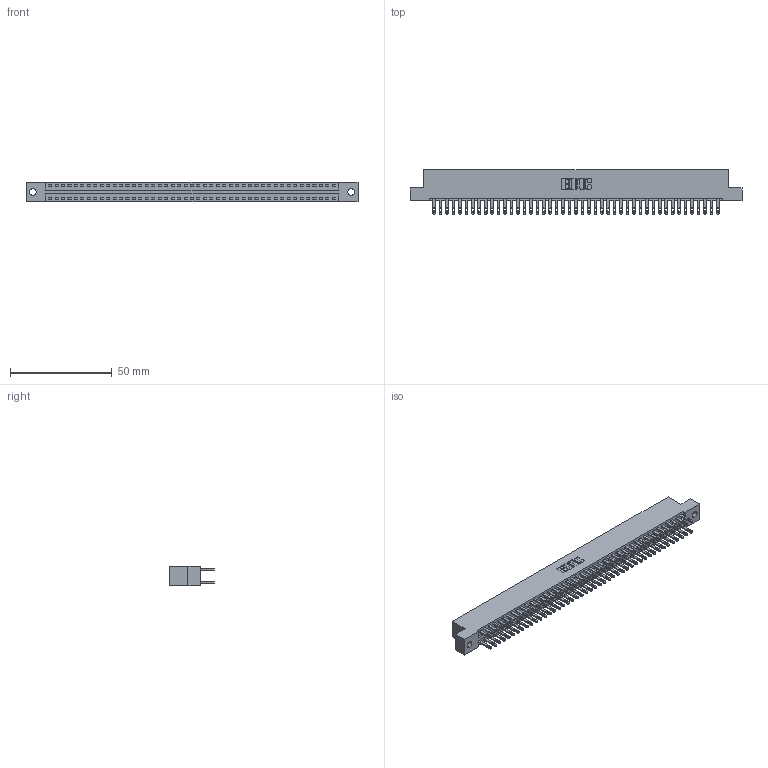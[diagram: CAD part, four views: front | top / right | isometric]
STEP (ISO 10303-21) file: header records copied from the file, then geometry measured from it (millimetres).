
FILE_DESCRIPTION (( 'STEP AP203' ), '1' );
FILE_NAME ('896-090-500-202.STEP', '2021-07-28T02:50:37', ( '' ), ( '' ), 'SwSTEP 2.0', 'SolidWorks 2020', '' );
FILE_SCHEMA (( 'CONFIG_CONTROL_DESIGN' ));
Length unit declared in the file: inch
Products named in the file (3): 846 Part_Flush Mounting Lugs - 0.128 Dia; 345-292-001_345-293-100; 896-090-500-202
Assembly tree (91 placements, depth 2):
  896-090-500-202
    846 Part_Flush Mounting Lugs - 0.128 Dia
    345-292-001_345-293-100  x90
Bounding box: 163.45 x 21.84 x 9.4 mm (x, y, z)
Volume: 16199.9 mm3; surface area: 22987.8 mm2
Topology: 91 solids, 91 shells, 4442 faces, 13559 edges, 9038 vertices
Faces by surface type: plane 2686, cylinder 1756
Entity records: 28897 total; most frequent: CARTESIAN_POINT 4756, ORIENTED_EDGE 4690, DIRECTION 4245, EDGE_CURVE 2345, VECTOR 2029, LINE 2029, VERTEX_POINT 1562, AXIS2_PLACEMENT_3D 1108
